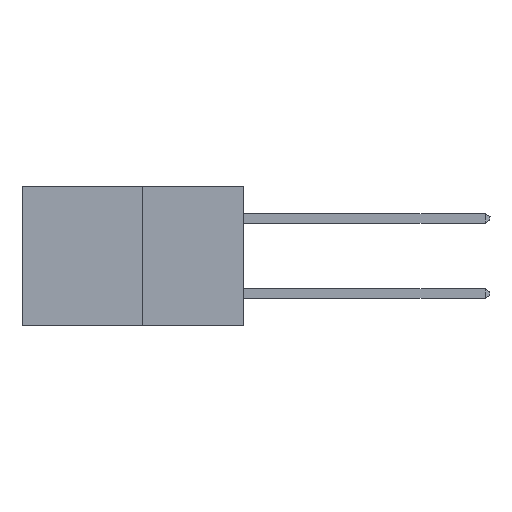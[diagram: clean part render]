
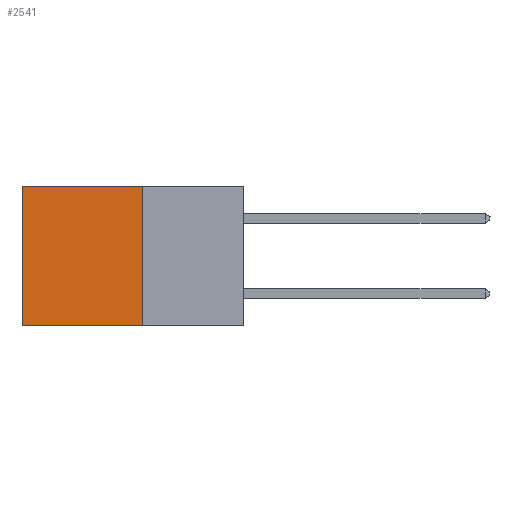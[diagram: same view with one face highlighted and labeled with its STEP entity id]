
A CAD part, left-side view. The second image highlights one B-rep face of the part: STEP entity #2541.
In plain terms, the highlighted planar face has unit normal (-1, 0, 0).
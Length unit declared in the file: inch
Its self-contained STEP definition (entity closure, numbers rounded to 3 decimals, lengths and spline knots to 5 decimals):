
#45 = VERTEX_POINT ( 'NONE', #1962 ) ;
#200 = ORIENTED_EDGE ( 'NONE', *, *, #4303, .F. ) ;
#278 = VECTOR ( 'NONE', #695, 39.37008 ) ;
#334 = CARTESIAN_POINT ( 'NONE',  ( 0.277, 0.59, 0. ) ) ;
#448 = CARTESIAN_POINT ( 'NONE',  ( 0.277, 0.27, -0.37 ) ) ;
#695 = DIRECTION ( 'NONE',  ( 0., 1., 0. ) ) ;
#862 = DIRECTION ( 'NONE',  ( 0., 0., -1. ) ) ;
#1104 = LINE ( 'NONE', #4674, #4760 ) ;
#1685 = DIRECTION ( 'NONE',  ( 0., 1., 0. ) ) ;
#1810 = CARTESIAN_POINT ( 'NONE',  ( 0.277, 0.27, -0.37 ) ) ;
#1867 = LINE ( 'NONE', #1810, #5451 ) ;
#1962 = CARTESIAN_POINT ( 'NONE',  ( 0.277, 0.27, 0. ) ) ;
#2126 = ORIENTED_EDGE ( 'NONE', *, *, #5341, .F. ) ;
#2407 = EDGE_LOOP ( 'NONE', ( #7436, #200, #2126, #4094 ) ) ;
#2541 = ADVANCED_FACE ( 'NONE', ( #7920 ), #7038, .F. ) ;
#4094 = ORIENTED_EDGE ( 'NONE', *, *, #4496, .T. ) ;
#4303 = EDGE_CURVE ( 'NONE', #4406, #6775, #1867, .T. ) ;
#4406 = VERTEX_POINT ( 'NONE', #448 ) ;
#4496 = EDGE_CURVE ( 'NONE', #45, #5837, #6162, .T. ) ;
#4659 = CARTESIAN_POINT ( 'NONE',  ( 0.277, 0.27, 0. ) ) ;
#4674 = CARTESIAN_POINT ( 'NONE',  ( 0.277, 0.59, -0.37 ) ) ;
#4760 = VECTOR ( 'NONE', #5794, 39.37008 ) ;
#4911 = DIRECTION ( 'NONE',  ( 1., 0., 0. ) ) ;
#5326 = VECTOR ( 'NONE', #5613, 39.37008 ) ;
#5341 = EDGE_CURVE ( 'NONE', #45, #4406, #7075, .T. ) ;
#5451 = VECTOR ( 'NONE', #1685, 39.37008 ) ;
#5613 = DIRECTION ( 'NONE',  ( 0., 0., -1. ) ) ;
#5761 = CARTESIAN_POINT ( 'NONE',  ( 0.277, 0.27, -0.37 ) ) ;
#5794 = DIRECTION ( 'NONE',  ( 0., 0., -1. ) ) ;
#5837 = VERTEX_POINT ( 'NONE', #334 ) ;
#6162 = LINE ( 'NONE', #4659, #278 ) ;
#6442 = CARTESIAN_POINT ( 'NONE',  ( 0.277, 0.59, -0.37 ) ) ;
#6775 = VERTEX_POINT ( 'NONE', #6442 ) ;
#7038 = PLANE ( 'NONE',  #8088 ) ;
#7056 = EDGE_CURVE ( 'NONE', #5837, #6775, #1104, .T. ) ;
#7075 = LINE ( 'NONE', #5761, #5326 ) ;
#7436 = ORIENTED_EDGE ( 'NONE', *, *, #7056, .T. ) ;
#7920 = FACE_OUTER_BOUND ( 'NONE', #2407, .T. ) ;
#8088 = AXIS2_PLACEMENT_3D ( 'NONE', #8582, #4911, #862 ) ;
#8582 = CARTESIAN_POINT ( 'NONE',  ( 0.277, 0.27, -0.37 ) ) ;
